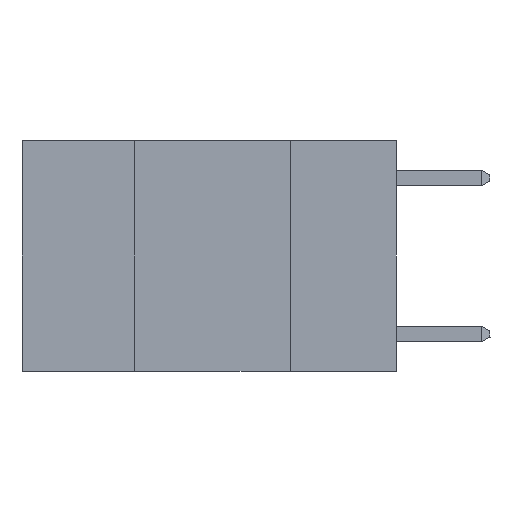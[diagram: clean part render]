
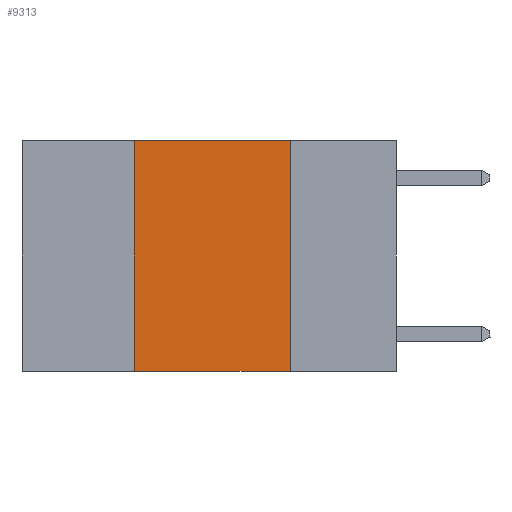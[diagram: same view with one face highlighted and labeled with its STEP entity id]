
A CAD part, left-side view. The second image highlights one B-rep face of the part: STEP entity #9313.
In plain terms, the highlighted planar face has unit normal (-1, 0, 0).
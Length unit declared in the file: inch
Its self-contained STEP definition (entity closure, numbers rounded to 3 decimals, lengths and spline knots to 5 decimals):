
#44 = DIRECTION ( 'NONE',  ( 1., 0., 0. ) ) ;
#1244 = AXIS2_PLACEMENT_3D ( 'NONE', #10713, #44, #6419 ) ;
#1414 = VECTOR ( 'NONE', #6166, 39.37008 ) ;
#1570 = VERTEX_POINT ( 'NONE', #5795 ) ;
#1637 = EDGE_CURVE ( 'NONE', #11183, #7691, #10717, .T. ) ;
#1714 = EDGE_CURVE ( 'NONE', #8615, #1570, #4381, .T. ) ;
#1768 = EDGE_CURVE ( 'NONE', #8615, #7691, #3836, .T. ) ;
#1997 = VECTOR ( 'NONE', #10409, 39.37008 ) ;
#2703 = CARTESIAN_POINT ( 'NONE',  ( 0., 0.17, 0. ) ) ;
#2927 = ORIENTED_EDGE ( 'NONE', *, *, #1637, .F. ) ;
#3033 = ORIENTED_EDGE ( 'NONE', *, *, #8940, .F. ) ;
#3081 = ORIENTED_EDGE ( 'NONE', *, *, #1714, .F. ) ;
#3126 = ORIENTED_EDGE ( 'NONE', *, *, #1768, .T. ) ;
#3818 = VECTOR ( 'NONE', #5032, 39.37008 ) ;
#3836 = LINE ( 'NONE', #10494, #1414 ) ;
#4381 = LINE ( 'NONE', #6937, #1997 ) ;
#4580 = PLANE ( 'NONE',  #1244 ) ;
#4990 = CARTESIAN_POINT ( 'NONE',  ( 0., 0.17, 0. ) ) ;
#5032 = DIRECTION ( 'NONE',  ( 0., -1., 0. ) ) ;
#5795 = CARTESIAN_POINT ( 'NONE',  ( 0., 0.42, 0. ) ) ;
#5936 = LINE ( 'NONE', #10269, #3818 ) ;
#6166 = DIRECTION ( 'NONE',  ( 0., -1., 0. ) ) ;
#6419 = DIRECTION ( 'NONE',  ( 0., 0., -1. ) ) ;
#6685 = CARTESIAN_POINT ( 'NONE',  ( 0., 0.17, -0.37 ) ) ;
#6937 = CARTESIAN_POINT ( 'NONE',  ( 0., 0.42, 0. ) ) ;
#7379 = CARTESIAN_POINT ( 'NONE',  ( 0., 0.42, -0.37 ) ) ;
#7691 = VERTEX_POINT ( 'NONE', #6685 ) ;
#8180 = VECTOR ( 'NONE', #9421, 39.37008 ) ;
#8615 = VERTEX_POINT ( 'NONE', #7379 ) ;
#8940 = EDGE_CURVE ( 'NONE', #1570, #11183, #5936, .T. ) ;
#9103 = FACE_OUTER_BOUND ( 'NONE', #10943, .T. ) ;
#9313 = ADVANCED_FACE ( 'NONE', ( #9103 ), #4580, .F. ) ;
#9421 = DIRECTION ( 'NONE',  ( 0., 0., -1. ) ) ;
#10269 = CARTESIAN_POINT ( 'NONE',  ( 0., 0.6, 0. ) ) ;
#10409 = DIRECTION ( 'NONE',  ( 0., 0., 1. ) ) ;
#10494 = CARTESIAN_POINT ( 'NONE',  ( 0., 0.6, -0.37 ) ) ;
#10713 = CARTESIAN_POINT ( 'NONE',  ( 0., 0.6, 0. ) ) ;
#10717 = LINE ( 'NONE', #4990, #8180 ) ;
#10943 = EDGE_LOOP ( 'NONE', ( #2927, #3033, #3081, #3126 ) ) ;
#11183 = VERTEX_POINT ( 'NONE', #2703 ) ;
